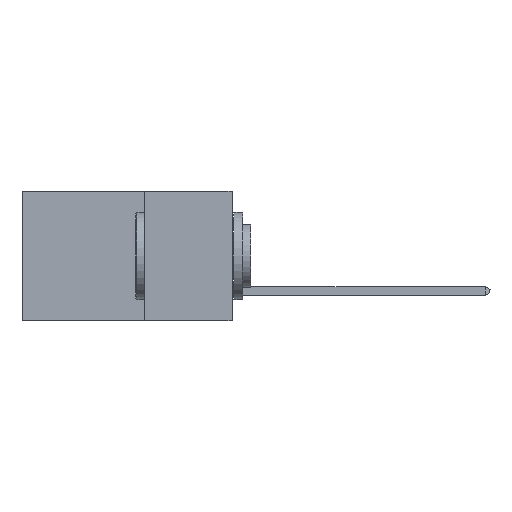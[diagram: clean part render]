
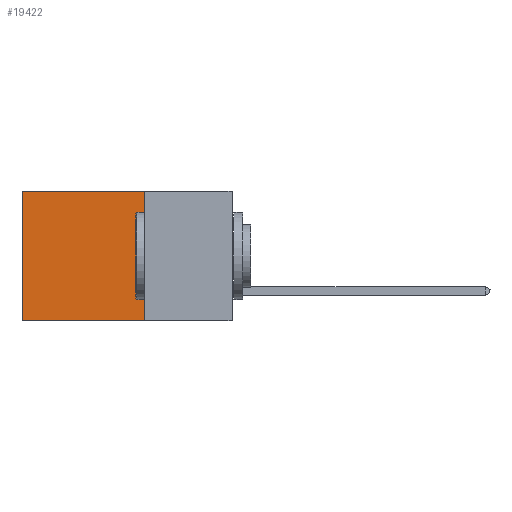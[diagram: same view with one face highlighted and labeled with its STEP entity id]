
A CAD part, left-side view. The second image highlights one B-rep face of the part: STEP entity #19422.
In plain terms, the highlighted planar face has unit normal (-1, 0, 0).
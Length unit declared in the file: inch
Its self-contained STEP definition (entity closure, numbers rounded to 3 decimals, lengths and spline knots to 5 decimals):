
#1281 = DIRECTION ( 'NONE',  ( 0., 0., -1. ) ) ;
#1661 = VERTEX_POINT ( 'NONE', #5336 ) ;
#2995 = ORIENTED_EDGE ( 'NONE', *, *, #3054, .T. ) ;
#3054 = EDGE_CURVE ( 'NONE', #1661, #12113, #18557, .T. ) ;
#3609 = LINE ( 'NONE', #7703, #4474 ) ;
#3942 = CARTESIAN_POINT ( 'NONE',  ( 0.2875, 0.6, 0. ) ) ;
#4474 = VECTOR ( 'NONE', #9640, 39.37008 ) ;
#5336 = CARTESIAN_POINT ( 'NONE',  ( 0.2875, 0.25, 0. ) ) ;
#5640 = EDGE_LOOP ( 'NONE', ( #14085, #7372, #12747, #2995 ) ) ;
#5919 = AXIS2_PLACEMENT_3D ( 'NONE', #11439, #5961, #1281 ) ;
#5961 = DIRECTION ( 'NONE',  ( 1., 0., 0. ) ) ;
#6020 = DIRECTION ( 'NONE',  ( 0., 0., -1. ) ) ;
#6521 = CARTESIAN_POINT ( 'NONE',  ( 0.2875, 0.6, 0. ) ) ;
#7372 = ORIENTED_EDGE ( 'NONE', *, *, #15418, .F. ) ;
#7703 = CARTESIAN_POINT ( 'NONE',  ( 0.2875, 0.25, -0.37 ) ) ;
#8446 = FACE_OUTER_BOUND ( 'NONE', #5640, .T. ) ;
#8881 = LINE ( 'NONE', #3942, #18353 ) ;
#9175 = CARTESIAN_POINT ( 'NONE',  ( 0.2875, 0.25, 0. ) ) ;
#9640 = DIRECTION ( 'NONE',  ( 0., 1., 0. ) ) ;
#11439 = CARTESIAN_POINT ( 'NONE',  ( 0.2875, 0.25, 0. ) ) ;
#11604 = EDGE_CURVE ( 'NONE', #1661, #18787, #18141, .T. ) ;
#12087 = DIRECTION ( 'NONE',  ( 0., 0., -1. ) ) ;
#12113 = VERTEX_POINT ( 'NONE', #6521 ) ;
#12394 = EDGE_CURVE ( 'NONE', #12113, #14983, #8881, .T. ) ;
#12747 = ORIENTED_EDGE ( 'NONE', *, *, #11604, .F. ) ;
#13112 = VECTOR ( 'NONE', #6020, 39.37008 ) ;
#14085 = ORIENTED_EDGE ( 'NONE', *, *, #12394, .T. ) ;
#14983 = VERTEX_POINT ( 'NONE', #24620 ) ;
#15418 = EDGE_CURVE ( 'NONE', #18787, #14983, #3609, .T. ) ;
#15460 = CARTESIAN_POINT ( 'NONE',  ( 0.2875, 0.25, 0. ) ) ;
#16450 = DIRECTION ( 'NONE',  ( 0., 1., 0. ) ) ;
#17855 = CARTESIAN_POINT ( 'NONE',  ( 0.2875, 0.25, -0.37 ) ) ;
#18141 = LINE ( 'NONE', #15460, #13112 ) ;
#18353 = VECTOR ( 'NONE', #12087, 39.37008 ) ;
#18557 = LINE ( 'NONE', #9175, #24205 ) ;
#18787 = VERTEX_POINT ( 'NONE', #17855 ) ;
#19422 = ADVANCED_FACE ( 'NONE', ( #8446 ), #24171, .F. ) ;
#24171 = PLANE ( 'NONE',  #5919 ) ;
#24205 = VECTOR ( 'NONE', #16450, 39.37008 ) ;
#24620 = CARTESIAN_POINT ( 'NONE',  ( 0.2875, 0.6, -0.37 ) ) ;
